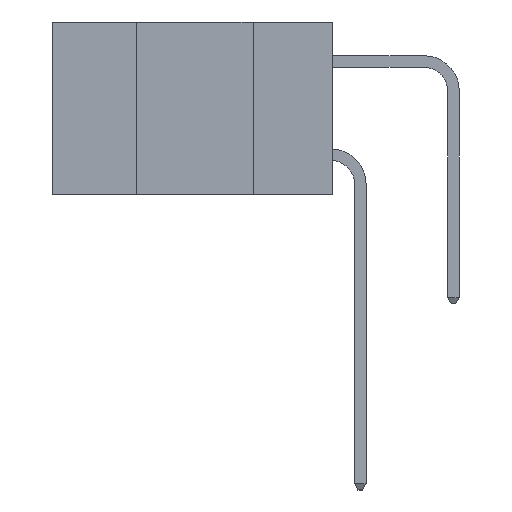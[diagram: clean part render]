
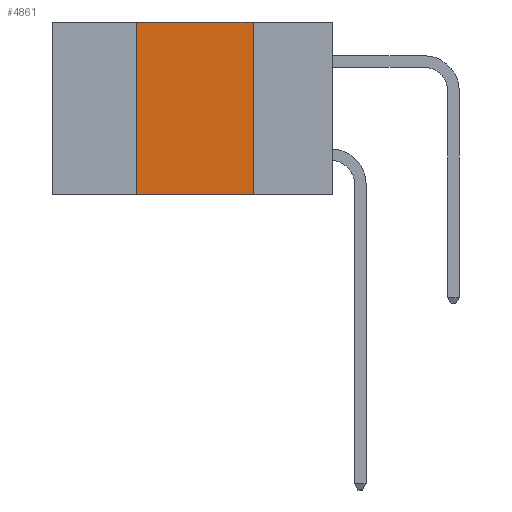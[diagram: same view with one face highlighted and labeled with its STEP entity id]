
A CAD part, left-side view. The second image highlights one B-rep face of the part: STEP entity #4861.
In plain terms, the highlighted planar face has unit normal (-1, 0, 0).
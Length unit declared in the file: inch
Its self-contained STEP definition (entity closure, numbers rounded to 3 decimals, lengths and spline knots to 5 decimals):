
#274 = LINE ( 'NONE', #7960, #12772 ) ;
#390 = ORIENTED_EDGE ( 'NONE', *, *, #6847, .F. ) ;
#922 = ORIENTED_EDGE ( 'NONE', *, *, #9828, .F. ) ;
#1297 = CARTESIAN_POINT ( 'NONE',  ( 0., 0.42, -0.37 ) ) ;
#1481 = LINE ( 'NONE', #12956, #10525 ) ;
#2178 = EDGE_CURVE ( 'NONE', #18731, #5045, #15994, .T. ) ;
#3865 = ORIENTED_EDGE ( 'NONE', *, *, #17499, .F. ) ;
#4861 = ADVANCED_FACE ( 'NONE', ( #12300 ), #17178, .F. ) ;
#5045 = VERTEX_POINT ( 'NONE', #15999 ) ;
#5322 = CARTESIAN_POINT ( 'NONE',  ( 0., 0.42, 0. ) ) ;
#5804 = AXIS2_PLACEMENT_3D ( 'NONE', #12090, #20576, #10437 ) ;
#6847 = EDGE_CURVE ( 'NONE', #17739, #15967, #274, .T. ) ;
#6949 = VECTOR ( 'NONE', #20525, 39.37008 ) ;
#7960 = CARTESIAN_POINT ( 'NONE',  ( 0., 0.6, 0. ) ) ;
#8612 = VECTOR ( 'NONE', #19912, 39.37008 ) ;
#9692 = LINE ( 'NONE', #1297, #8612 ) ;
#9828 = EDGE_CURVE ( 'NONE', #18731, #17739, #9692, .T. ) ;
#10384 = CARTESIAN_POINT ( 'NONE',  ( 0., 0.6, -0.37 ) ) ;
#10437 = DIRECTION ( 'NONE',  ( 0., 0., -1. ) ) ;
#10525 = VECTOR ( 'NONE', #14654, 39.37008 ) ;
#12090 = CARTESIAN_POINT ( 'NONE',  ( 0., 0.6, 0. ) ) ;
#12300 = FACE_OUTER_BOUND ( 'NONE', #16997, .T. ) ;
#12772 = VECTOR ( 'NONE', #21512, 39.37008 ) ;
#12956 = CARTESIAN_POINT ( 'NONE',  ( 0., 0.17, -0.37 ) ) ;
#14654 = DIRECTION ( 'NONE',  ( 0., 0., -1. ) ) ;
#15690 = CARTESIAN_POINT ( 'NONE',  ( 0., 0.17, 0. ) ) ;
#15967 = VERTEX_POINT ( 'NONE', #15690 ) ;
#15994 = LINE ( 'NONE', #10384, #6949 ) ;
#15999 = CARTESIAN_POINT ( 'NONE',  ( 0., 0.17, -0.37 ) ) ;
#16997 = EDGE_LOOP ( 'NONE', ( #3865, #390, #922, #17116 ) ) ;
#17116 = ORIENTED_EDGE ( 'NONE', *, *, #2178, .T. ) ;
#17178 = PLANE ( 'NONE',  #5804 ) ;
#17499 = EDGE_CURVE ( 'NONE', #15967, #5045, #1481, .T. ) ;
#17739 = VERTEX_POINT ( 'NONE', #5322 ) ;
#18731 = VERTEX_POINT ( 'NONE', #21340 ) ;
#19912 = DIRECTION ( 'NONE',  ( 0., 0., 1. ) ) ;
#20525 = DIRECTION ( 'NONE',  ( 0., -1., 0. ) ) ;
#20576 = DIRECTION ( 'NONE',  ( 1., 0., 0. ) ) ;
#21340 = CARTESIAN_POINT ( 'NONE',  ( 0., 0.42, -0.37 ) ) ;
#21512 = DIRECTION ( 'NONE',  ( 0., -1., 0. ) ) ;
